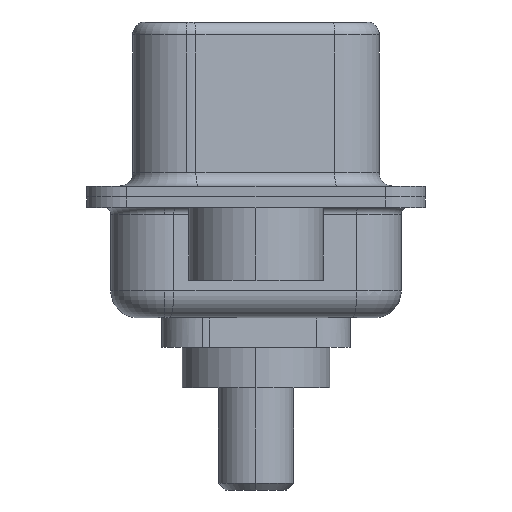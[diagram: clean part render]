
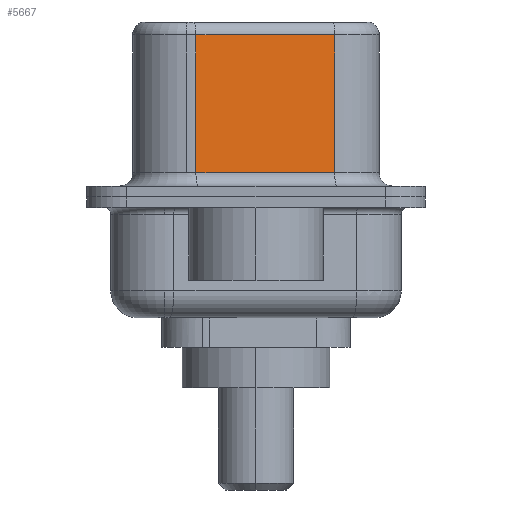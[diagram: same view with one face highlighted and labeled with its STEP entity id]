
A CAD part, left-side view. The second image highlights one B-rep face of the part: STEP entity #5667.
In plain terms, the highlighted planar face has unit normal (-0.985, -0.174, 0).
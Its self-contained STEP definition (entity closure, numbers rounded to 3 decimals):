
#381 = VERTEX_POINT ( 'NONE', #11098 ) ;
#763 = CARTESIAN_POINT ( 'NONE',  ( 4.565, -2.927, 0.9 ) ) ;
#1074 = DIRECTION ( 'NONE',  ( 0., 0., -1. ) ) ;
#1602 = ORIENTED_EDGE ( 'NONE', *, *, #1854, .F. ) ;
#1854 = EDGE_CURVE ( 'NONE', #11753, #381, #9525, .T. ) ;
#2336 = CARTESIAN_POINT ( 'NONE',  ( 4.565, -2.927, 6.02 ) ) ;
#3026 = DIRECTION ( 'NONE',  ( 0.985, 0.174, 0. ) ) ;
#3249 = ORIENTED_EDGE ( 'NONE', *, *, #6635, .T. ) ;
#3906 = CARTESIAN_POINT ( 'NONE',  ( 4.565, -2.927, 6.52 ) ) ;
#4473 = EDGE_LOOP ( 'NONE', ( #1602, #7912, #9989, #3249 ) ) ;
#4904 = CARTESIAN_POINT ( 'NONE',  ( 4.565, -2.927, 6.52 ) ) ;
#5171 = VECTOR ( 'NONE', #12573, 1000. ) ;
#5511 = DIRECTION ( 'NONE',  ( -0.174, 0.985, 0. ) ) ;
#5597 = VERTEX_POINT ( 'NONE', #10377 ) ;
#5667 = ADVANCED_FACE ( 'NONE', ( #6014 ), #7574, .F. ) ;
#6014 = FACE_OUTER_BOUND ( 'NONE', #4473, .T. ) ;
#6559 = EDGE_CURVE ( 'NONE', #9382, #5597, #8363, .T. ) ;
#6635 = EDGE_CURVE ( 'NONE', #5597, #381, #7800, .T. ) ;
#6696 = VECTOR ( 'NONE', #12736, 1000. ) ;
#7169 = VECTOR ( 'NONE', #10450, 1000. ) ;
#7574 = PLANE ( 'NONE',  #11871 ) ;
#7675 = CARTESIAN_POINT ( 'NONE',  ( 3.655, 2.233, 6.52 ) ) ;
#7800 = LINE ( 'NONE', #763, #5171 ) ;
#7912 = ORIENTED_EDGE ( 'NONE', *, *, #9641, .T. ) ;
#8363 = LINE ( 'NONE', #7675, #10983 ) ;
#9382 = VERTEX_POINT ( 'NONE', #10686 ) ;
#9525 = LINE ( 'NONE', #4904, #6696 ) ;
#9641 = EDGE_CURVE ( 'NONE', #11753, #9382, #9700, .T. ) ;
#9700 = LINE ( 'NONE', #10581, #7169 ) ;
#9989 = ORIENTED_EDGE ( 'NONE', *, *, #6559, .T. ) ;
#10377 = CARTESIAN_POINT ( 'NONE',  ( 3.655, 2.233, 0.9 ) ) ;
#10450 = DIRECTION ( 'NONE',  ( -0.174, 0.985, 0. ) ) ;
#10581 = CARTESIAN_POINT ( 'NONE',  ( 4.565, -2.927, 6.02 ) ) ;
#10686 = CARTESIAN_POINT ( 'NONE',  ( 3.655, 2.233, 6.02 ) ) ;
#10983 = VECTOR ( 'NONE', #1074, 1000. ) ;
#11098 = CARTESIAN_POINT ( 'NONE',  ( 4.565, -2.927, 0.9 ) ) ;
#11753 = VERTEX_POINT ( 'NONE', #2336 ) ;
#11871 = AXIS2_PLACEMENT_3D ( 'NONE', #3906, #3026, #5511 ) ;
#12573 = DIRECTION ( 'NONE',  ( 0.174, -0.985, 0. ) ) ;
#12736 = DIRECTION ( 'NONE',  ( 0., 0., -1. ) ) ;
